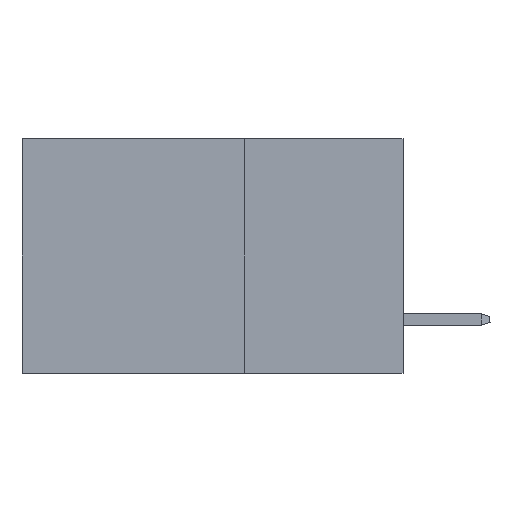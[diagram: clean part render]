
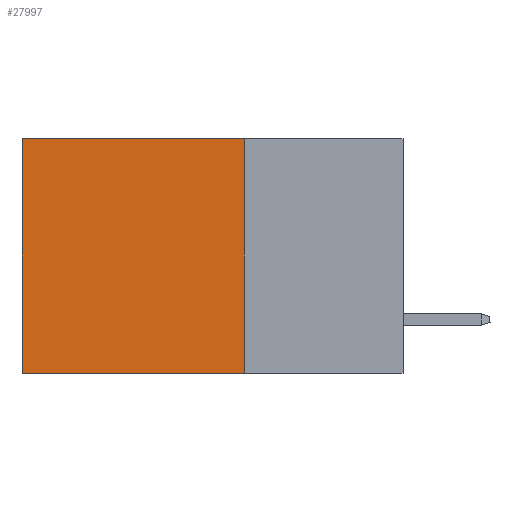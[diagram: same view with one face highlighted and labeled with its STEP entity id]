
A CAD part, left-side view. The second image highlights one B-rep face of the part: STEP entity #27997.
In plain terms, the highlighted planar face has unit normal (-1, 0, 0).
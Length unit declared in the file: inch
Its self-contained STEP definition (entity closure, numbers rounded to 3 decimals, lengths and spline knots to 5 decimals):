
#726 = VECTOR ( 'NONE', #22193, 39.37008 ) ;
#1330 = EDGE_CURVE ( 'NONE', #1677, #29073, #7336, .T. ) ;
#1677 = VERTEX_POINT ( 'NONE', #17685 ) ;
#4895 = CARTESIAN_POINT ( 'NONE',  ( 0.2875, 0.25, 0. ) ) ;
#6953 = CARTESIAN_POINT ( 'NONE',  ( 0.2875, 0.25, -0.37 ) ) ;
#7336 = LINE ( 'NONE', #31226, #8221 ) ;
#7507 = DIRECTION ( 'NONE',  ( 0., 0., -1. ) ) ;
#7663 = DIRECTION ( 'NONE',  ( 0., 1., 0. ) ) ;
#8015 = ORIENTED_EDGE ( 'NONE', *, *, #1330, .T. ) ;
#8221 = VECTOR ( 'NONE', #7507, 39.37008 ) ;
#9470 = VERTEX_POINT ( 'NONE', #4895 ) ;
#14056 = LINE ( 'NONE', #24625, #726 ) ;
#14457 = VECTOR ( 'NONE', #30704, 39.37008 ) ;
#14957 = LINE ( 'NONE', #23250, #14457 ) ;
#17321 = ORIENTED_EDGE ( 'NONE', *, *, #31854, .T. ) ;
#17685 = CARTESIAN_POINT ( 'NONE',  ( 0.2875, 0.6, 0. ) ) ;
#18017 = EDGE_CURVE ( 'NONE', #29029, #29073, #20988, .T. ) ;
#18679 = PLANE ( 'NONE',  #20421 ) ;
#18722 = CARTESIAN_POINT ( 'NONE',  ( 0.2875, 0.25, -0.37 ) ) ;
#20421 = AXIS2_PLACEMENT_3D ( 'NONE', #24047, #20781, #28576 ) ;
#20572 = ORIENTED_EDGE ( 'NONE', *, *, #33590, .F. ) ;
#20781 = DIRECTION ( 'NONE',  ( 1., 0., 0. ) ) ;
#20917 = ORIENTED_EDGE ( 'NONE', *, *, #18017, .F. ) ;
#20988 = LINE ( 'NONE', #18722, #26617 ) ;
#21457 = EDGE_LOOP ( 'NONE', ( #8015, #20917, #20572, #17321 ) ) ;
#22193 = DIRECTION ( 'NONE',  ( 0., 0., -1. ) ) ;
#22527 = CARTESIAN_POINT ( 'NONE',  ( 0.2875, 0.6, -0.37 ) ) ;
#23250 = CARTESIAN_POINT ( 'NONE',  ( 0.2875, 0.25, 0. ) ) ;
#24047 = CARTESIAN_POINT ( 'NONE',  ( 0.2875, 0.25, 0. ) ) ;
#24625 = CARTESIAN_POINT ( 'NONE',  ( 0.2875, 0.25, 0. ) ) ;
#26617 = VECTOR ( 'NONE', #7663, 39.37008 ) ;
#27997 = ADVANCED_FACE ( 'NONE', ( #29239 ), #18679, .F. ) ;
#28576 = DIRECTION ( 'NONE',  ( 0., 0., -1. ) ) ;
#29029 = VERTEX_POINT ( 'NONE', #6953 ) ;
#29073 = VERTEX_POINT ( 'NONE', #22527 ) ;
#29239 = FACE_OUTER_BOUND ( 'NONE', #21457, .T. ) ;
#30704 = DIRECTION ( 'NONE',  ( 0., 1., 0. ) ) ;
#31226 = CARTESIAN_POINT ( 'NONE',  ( 0.2875, 0.6, 0. ) ) ;
#31854 = EDGE_CURVE ( 'NONE', #9470, #1677, #14957, .T. ) ;
#33590 = EDGE_CURVE ( 'NONE', #9470, #29029, #14056, .T. ) ;
